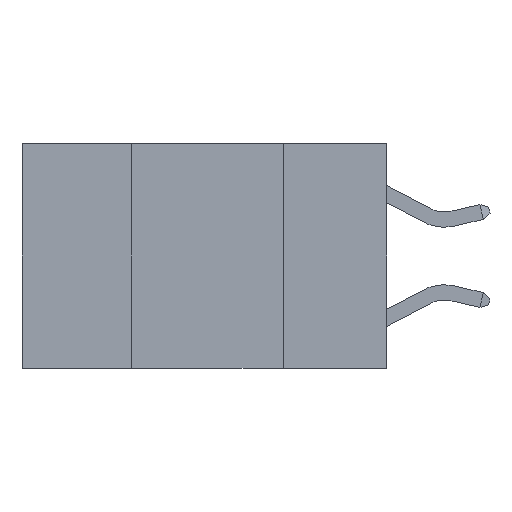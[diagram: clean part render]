
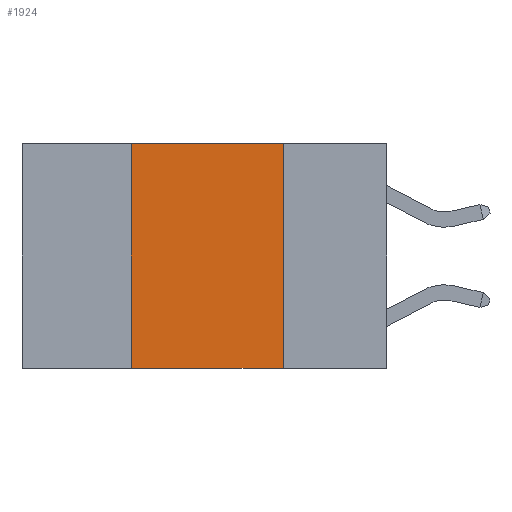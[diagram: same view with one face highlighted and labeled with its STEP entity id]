
A CAD part, left-side view. The second image highlights one B-rep face of the part: STEP entity #1924.
In plain terms, the highlighted planar face has unit normal (-1, 0, 0).
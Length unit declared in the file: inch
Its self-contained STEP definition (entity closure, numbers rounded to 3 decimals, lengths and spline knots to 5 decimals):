
#103 = VERTEX_POINT ( 'NONE', #7769 ) ;
#175 = VECTOR ( 'NONE', #3212, 39.37008 ) ;
#1553 = VECTOR ( 'NONE', #4516, 39.37008 ) ;
#1802 = VECTOR ( 'NONE', #5253, 39.37008 ) ;
#1924 = ADVANCED_FACE ( 'NONE', ( #4998 ), #9602, .F. ) ;
#2364 = DIRECTION ( 'NONE',  ( 1., 0., 0. ) ) ;
#3149 = ORIENTED_EDGE ( 'NONE', *, *, #7807, .T. ) ;
#3212 = DIRECTION ( 'NONE',  ( 0., -1., 0. ) ) ;
#3662 = LINE ( 'NONE', #9058, #1802 ) ;
#3819 = CARTESIAN_POINT ( 'NONE',  ( 0., 0.42, 0. ) ) ;
#3881 = LINE ( 'NONE', #9657, #5578 ) ;
#3952 = CARTESIAN_POINT ( 'NONE',  ( 0., 0.6, 0. ) ) ;
#4516 = DIRECTION ( 'NONE',  ( 0., 0., 1. ) ) ;
#4561 = LINE ( 'NONE', #6163, #175 ) ;
#4771 = ORIENTED_EDGE ( 'NONE', *, *, #7791, .F. ) ;
#4998 = FACE_OUTER_BOUND ( 'NONE', #8738, .T. ) ;
#5083 = AXIS2_PLACEMENT_3D ( 'NONE', #3952, #2364, #9150 ) ;
#5253 = DIRECTION ( 'NONE',  ( 0., -1., 0. ) ) ;
#5284 = ORIENTED_EDGE ( 'NONE', *, *, #6291, .F. ) ;
#5291 = VERTEX_POINT ( 'NONE', #7770 ) ;
#5578 = VECTOR ( 'NONE', #8352, 39.37008 ) ;
#6163 = CARTESIAN_POINT ( 'NONE',  ( 0., 0.6, 0. ) ) ;
#6291 = EDGE_CURVE ( 'NONE', #7787, #5291, #4561, .T. ) ;
#6733 = CARTESIAN_POINT ( 'NONE',  ( 0., 0.42, 0. ) ) ;
#7215 = ORIENTED_EDGE ( 'NONE', *, *, #7792, .F. ) ;
#7318 = CARTESIAN_POINT ( 'NONE',  ( 0., 0.17, -0.37 ) ) ;
#7639 = LINE ( 'NONE', #3819, #1553 ) ;
#7769 = CARTESIAN_POINT ( 'NONE',  ( 0., 0.42, -0.37 ) ) ;
#7770 = CARTESIAN_POINT ( 'NONE',  ( 0., 0.17, 0. ) ) ;
#7787 = VERTEX_POINT ( 'NONE', #6733 ) ;
#7791 = EDGE_CURVE ( 'NONE', #5291, #9202, #3881, .T. ) ;
#7792 = EDGE_CURVE ( 'NONE', #103, #7787, #7639, .T. ) ;
#7807 = EDGE_CURVE ( 'NONE', #103, #9202, #3662, .T. ) ;
#8352 = DIRECTION ( 'NONE',  ( 0., 0., -1. ) ) ;
#8738 = EDGE_LOOP ( 'NONE', ( #4771, #5284, #7215, #3149 ) ) ;
#9058 = CARTESIAN_POINT ( 'NONE',  ( 0., 0.6, -0.37 ) ) ;
#9150 = DIRECTION ( 'NONE',  ( 0., 0., -1. ) ) ;
#9202 = VERTEX_POINT ( 'NONE', #7318 ) ;
#9602 = PLANE ( 'NONE',  #5083 ) ;
#9657 = CARTESIAN_POINT ( 'NONE',  ( 0., 0.17, 0. ) ) ;
